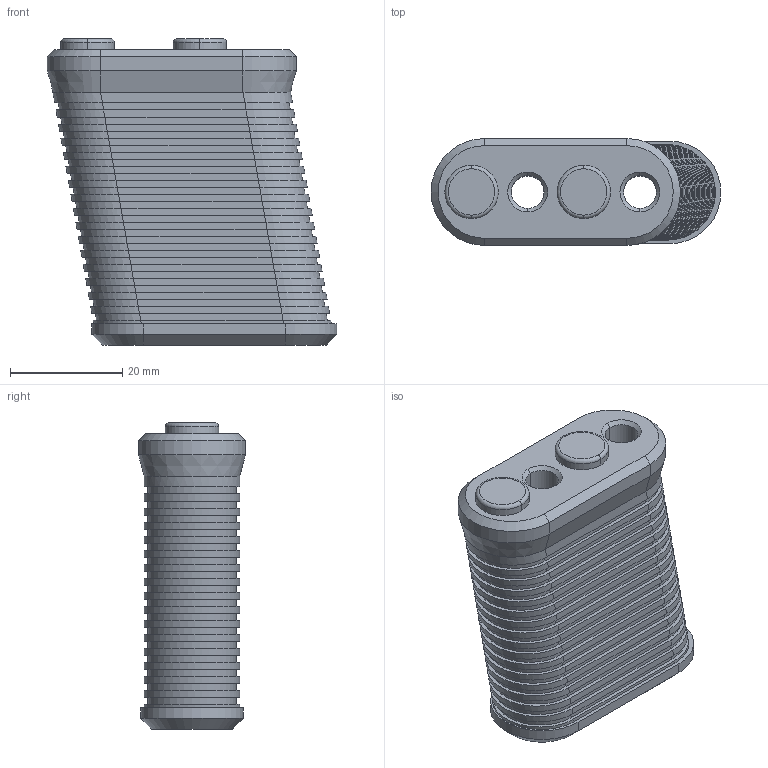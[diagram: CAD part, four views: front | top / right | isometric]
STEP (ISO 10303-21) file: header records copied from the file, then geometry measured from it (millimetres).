
FILE_DESCRIPTION (( 'STEP AP203' ), '1' );
FILE_NAME ('AF-WF-VF-PRT-001-STEP.STEP', '2020-07-22T01:03:37', ( '' ), ( '' ), 'SwSTEP 2.0', 'SolidWorks 2018', '' );
FILE_SCHEMA (( 'CONFIG_CONTROL_DESIGN' ));
Length unit declared in the file: inch
Products named in the file (1): AF-WF-VF-PRT-001-STEP
Bounding box: 51.68 x 19.05 x 54.61 mm (x, y, z)
Volume: 20722.5 mm3; surface area: 18462.7 mm2
Topology: 1 solids, 2 shells, 267 faces, 648 edges, 418 vertices
Faces by surface type: plane 153, bspline 68, cylinder 24, cone 18, torus 4
Entity records: 8184 total; most frequent: CARTESIAN_POINT 2183, ORIENTED_EDGE 1296, DIRECTION 1122, EDGE_CURVE 648, VERTEX_POINT 418, LINE 416, VECTOR 416, AXIS2_PLACEMENT_3D 353
